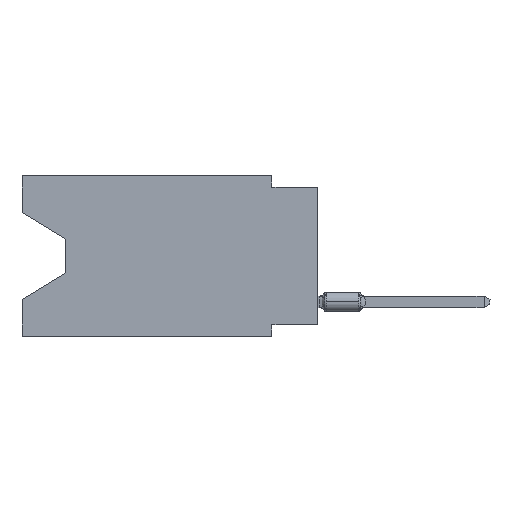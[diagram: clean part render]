
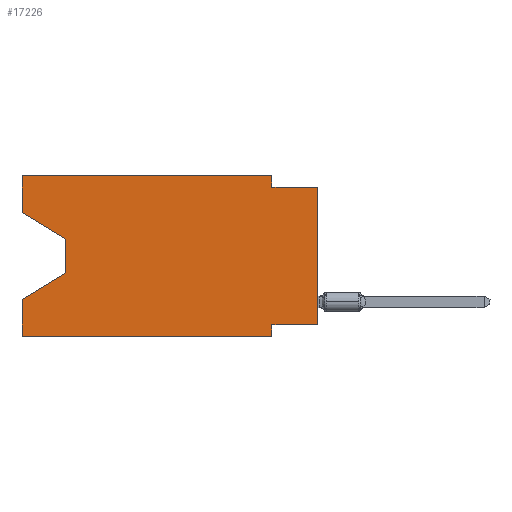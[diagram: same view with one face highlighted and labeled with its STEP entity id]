
A CAD part, left-side view. The second image highlights one B-rep face of the part: STEP entity #17226.
In plain terms, the highlighted planar face has unit normal (-1, 0, 0).
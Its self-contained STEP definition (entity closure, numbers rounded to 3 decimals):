
#592 = CARTESIAN_POINT ( 'NONE',  ( 0., 0., -8.255 ) ) ;
#1808 = VECTOR ( 'NONE', #24251, 1000. ) ;
#1819 = CARTESIAN_POINT ( 'NONE',  ( 0., 2.54, -8.89 ) ) ;
#1976 = CARTESIAN_POINT ( 'NONE',  ( 0., 16.383, -6.852 ) ) ;
#2040 = DIRECTION ( 'NONE',  ( 0., -1., 0. ) ) ;
#2214 = CARTESIAN_POINT ( 'NONE',  ( 0., 2.54, 0. ) ) ;
#3018 = ORIENTED_EDGE ( 'NONE', *, *, #24379, .T. ) ;
#3257 = VECTOR ( 'NONE', #6545, 1000. ) ;
#3407 = EDGE_CURVE ( 'NONE', #7988, #16032, #5838, .T. ) ;
#3977 = FACE_OUTER_BOUND ( 'NONE', #13625, .T. ) ;
#4567 = EDGE_CURVE ( 'NONE', #16032, #8997, #6966, .T. ) ;
#4705 = CARTESIAN_POINT ( 'NONE',  ( 0., 0., -0.635 ) ) ;
#4761 = ORIENTED_EDGE ( 'NONE', *, *, #18438, .T. ) ;
#4778 = CARTESIAN_POINT ( 'NONE',  ( 0., 16.383, 0. ) ) ;
#4855 = CARTESIAN_POINT ( 'NONE',  ( 0., 16.383, 0. ) ) ;
#5267 = VERTEX_POINT ( 'NONE', #21269 ) ;
#5446 = CARTESIAN_POINT ( 'NONE',  ( 0., 13.97, -5.385 ) ) ;
#5581 = LINE ( 'NONE', #8174, #7708 ) ;
#5838 = LINE ( 'NONE', #25871, #11066 ) ;
#6158 = VERTEX_POINT ( 'NONE', #4705 ) ;
#6545 = DIRECTION ( 'NONE',  ( 0., 0., -1. ) ) ;
#6755 = ORIENTED_EDGE ( 'NONE', *, *, #24999, .F. ) ;
#6885 = CARTESIAN_POINT ( 'NONE',  ( 0., 13.97, -3.505 ) ) ;
#6966 = LINE ( 'NONE', #22228, #3257 ) ;
#7548 = EDGE_CURVE ( 'NONE', #19691, #8439, #21817, .T. ) ;
#7708 = VECTOR ( 'NONE', #28058, 1000. ) ;
#7988 = VERTEX_POINT ( 'NONE', #592 ) ;
#8174 = CARTESIAN_POINT ( 'NONE',  ( 0., 16.383, 0. ) ) ;
#8191 = DIRECTION ( 'NONE',  ( 0., 0.855, -0.519 ) ) ;
#8427 = DIRECTION ( 'NONE',  ( 0., 0., 1. ) ) ;
#8439 = VERTEX_POINT ( 'NONE', #20161 ) ;
#8783 = EDGE_CURVE ( 'NONE', #11391, #5267, #10334, .T. ) ;
#8865 = LINE ( 'NONE', #26412, #23323 ) ;
#8868 = DIRECTION ( 'NONE',  ( 0., 0., -1. ) ) ;
#8997 = VERTEX_POINT ( 'NONE', #1819 ) ;
#9013 = VERTEX_POINT ( 'NONE', #15364 ) ;
#9090 = ORIENTED_EDGE ( 'NONE', *, *, #20255, .F. ) ;
#9260 = LINE ( 'NONE', #4778, #16892 ) ;
#9504 = ORIENTED_EDGE ( 'NONE', *, *, #16526, .T. ) ;
#9844 = VECTOR ( 'NONE', #13069, 1000. ) ;
#10070 = LINE ( 'NONE', #5446, #17977 ) ;
#10334 = LINE ( 'NONE', #2214, #18751 ) ;
#10735 = DIRECTION ( 'NONE',  ( 0., 0., 1. ) ) ;
#11066 = VECTOR ( 'NONE', #27876, 1000. ) ;
#11189 = DIRECTION ( 'NONE',  ( 0., 0., -1. ) ) ;
#11195 = LINE ( 'NONE', #11468, #27843 ) ;
#11256 = AXIS2_PLACEMENT_3D ( 'NONE', #20786, #18074, #11189 ) ;
#11391 = VERTEX_POINT ( 'NONE', #25469 ) ;
#11417 = EDGE_CURVE ( 'NONE', #8439, #24618, #10070, .T. ) ;
#11468 = CARTESIAN_POINT ( 'NONE',  ( 0., 16.383, -2.038 ) ) ;
#12775 = PLANE ( 'NONE',  #11256 ) ;
#13069 = DIRECTION ( 'NONE',  ( 0., -1., 0. ) ) ;
#13625 = EDGE_LOOP ( 'NONE', ( #4761, #20126, #16337, #6755, #9504, #20942, #23179, #3018, #9090, #16566, #18799, #18933 ) ) ;
#14359 = VECTOR ( 'NONE', #26882, 1000. ) ;
#14739 = EDGE_CURVE ( 'NONE', #20903, #11391, #18105, .T. ) ;
#15364 = CARTESIAN_POINT ( 'NONE',  ( 0., 16.383, -2.038 ) ) ;
#15462 = CARTESIAN_POINT ( 'NONE',  ( 0., 13.97, -3.505 ) ) ;
#16032 = VERTEX_POINT ( 'NONE', #23657 ) ;
#16337 = ORIENTED_EDGE ( 'NONE', *, *, #11417, .T. ) ;
#16526 = EDGE_CURVE ( 'NONE', #21512, #8997, #17361, .T. ) ;
#16566 = ORIENTED_EDGE ( 'NONE', *, *, #8783, .F. ) ;
#16892 = VECTOR ( 'NONE', #8427, 1000. ) ;
#17226 = ADVANCED_FACE ( 'NONE', ( #3977 ), #12775, .F. ) ;
#17361 = LINE ( 'NONE', #26167, #9844 ) ;
#17977 = VECTOR ( 'NONE', #8191, 1000. ) ;
#18074 = DIRECTION ( 'NONE',  ( 1., 0., 0. ) ) ;
#18088 = CARTESIAN_POINT ( 'NONE',  ( 0., 16.383, -8.89 ) ) ;
#18105 = LINE ( 'NONE', #4855, #14359 ) ;
#18438 = EDGE_CURVE ( 'NONE', #9013, #19691, #11195, .T. ) ;
#18751 = VECTOR ( 'NONE', #8868, 1000. ) ;
#18799 = ORIENTED_EDGE ( 'NONE', *, *, #14739, .F. ) ;
#18933 = ORIENTED_EDGE ( 'NONE', *, *, #25592, .F. ) ;
#19691 = VERTEX_POINT ( 'NONE', #6885 ) ;
#20126 = ORIENTED_EDGE ( 'NONE', *, *, #7548, .T. ) ;
#20161 = CARTESIAN_POINT ( 'NONE',  ( 0., 13.97, -5.385 ) ) ;
#20255 = EDGE_CURVE ( 'NONE', #5267, #6158, #23527, .T. ) ;
#20786 = CARTESIAN_POINT ( 'NONE',  ( 0., 16.383, 0. ) ) ;
#20903 = VERTEX_POINT ( 'NONE', #24096 ) ;
#20942 = ORIENTED_EDGE ( 'NONE', *, *, #4567, .F. ) ;
#21269 = CARTESIAN_POINT ( 'NONE',  ( 0., 2.54, -0.635 ) ) ;
#21512 = VERTEX_POINT ( 'NONE', #18088 ) ;
#21817 = LINE ( 'NONE', #15462, #1808 ) ;
#22228 = CARTESIAN_POINT ( 'NONE',  ( 0., 2.54, -8.89 ) ) ;
#23179 = ORIENTED_EDGE ( 'NONE', *, *, #3407, .F. ) ;
#23323 = VECTOR ( 'NONE', #10735, 1000. ) ;
#23527 = LINE ( 'NONE', #28126, #24017 ) ;
#23657 = CARTESIAN_POINT ( 'NONE',  ( 0., 2.54, -8.255 ) ) ;
#24017 = VECTOR ( 'NONE', #2040, 1000. ) ;
#24096 = CARTESIAN_POINT ( 'NONE',  ( 0., 16.383, 0. ) ) ;
#24251 = DIRECTION ( 'NONE',  ( 0., 0., -1. ) ) ;
#24296 = DIRECTION ( 'NONE',  ( 0., -0.855, -0.519 ) ) ;
#24379 = EDGE_CURVE ( 'NONE', #7988, #6158, #8865, .T. ) ;
#24618 = VERTEX_POINT ( 'NONE', #1976 ) ;
#24999 = EDGE_CURVE ( 'NONE', #21512, #24618, #9260, .T. ) ;
#25469 = CARTESIAN_POINT ( 'NONE',  ( 0., 2.54, 0. ) ) ;
#25592 = EDGE_CURVE ( 'NONE', #9013, #20903, #5581, .T. ) ;
#25871 = CARTESIAN_POINT ( 'NONE',  ( 0., 0., -8.255 ) ) ;
#26167 = CARTESIAN_POINT ( 'NONE',  ( 0., 16.383, -8.89 ) ) ;
#26412 = CARTESIAN_POINT ( 'NONE',  ( 0., 0., 0. ) ) ;
#26882 = DIRECTION ( 'NONE',  ( 0., -1., 0. ) ) ;
#27843 = VECTOR ( 'NONE', #24296, 1000. ) ;
#27876 = DIRECTION ( 'NONE',  ( 0., 1., 0. ) ) ;
#28058 = DIRECTION ( 'NONE',  ( 0., 0., 1. ) ) ;
#28126 = CARTESIAN_POINT ( 'NONE',  ( 0., 0., -0.635 ) ) ;
